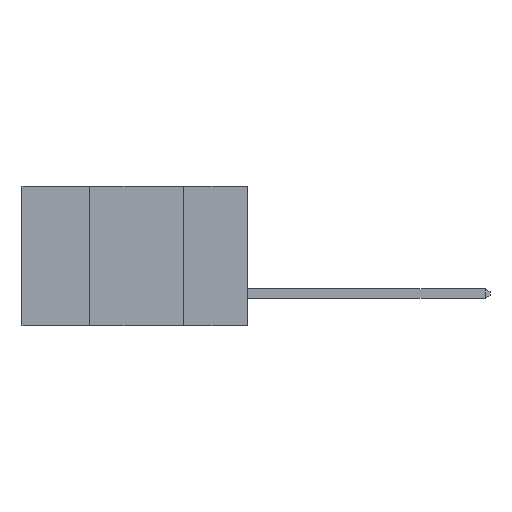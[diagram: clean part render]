
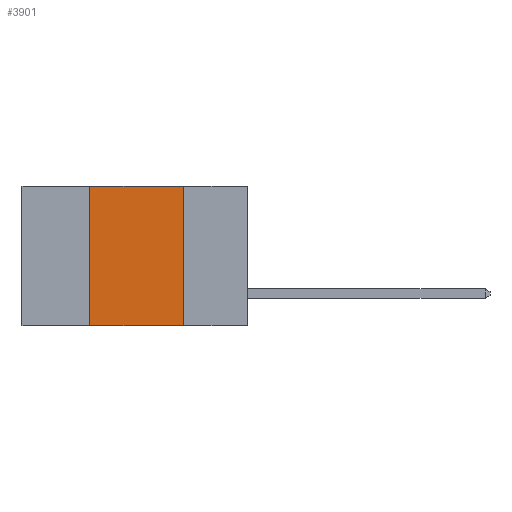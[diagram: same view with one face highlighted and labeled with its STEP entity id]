
A CAD part, left-side view. The second image highlights one B-rep face of the part: STEP entity #3901.
In plain terms, the highlighted planar face has unit normal (-1, 0, 0).
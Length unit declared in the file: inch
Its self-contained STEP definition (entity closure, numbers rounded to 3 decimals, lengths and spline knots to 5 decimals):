
#91 = CARTESIAN_POINT ( 'NONE',  ( 0., 0.6, -0.37 ) ) ;
#471 = CARTESIAN_POINT ( 'NONE',  ( 0., 0.6, 0. ) ) ;
#541 = EDGE_CURVE ( 'NONE', #9583, #4215, #10772, .T. ) ;
#1149 = LINE ( 'NONE', #91, #6142 ) ;
#1496 = ORIENTED_EDGE ( 'NONE', *, *, #4192, .T. ) ;
#2065 = LINE ( 'NONE', #2553, #7037 ) ;
#2484 = VECTOR ( 'NONE', #10289, 39.37008 ) ;
#2553 = CARTESIAN_POINT ( 'NONE',  ( 0., 0.42, 0. ) ) ;
#2764 = VERTEX_POINT ( 'NONE', #6121 ) ;
#2808 = LINE ( 'NONE', #4328, #5478 ) ;
#3460 = CARTESIAN_POINT ( 'NONE',  ( 0., 0.42, 0. ) ) ;
#3813 = EDGE_LOOP ( 'NONE', ( #11535, #6487, #9145, #1496 ) ) ;
#3901 = ADVANCED_FACE ( 'NONE', ( #4592 ), #4044, .F. ) ;
#3959 = AXIS2_PLACEMENT_3D ( 'NONE', #6208, #8726, #5074 ) ;
#4044 = PLANE ( 'NONE',  #3959 ) ;
#4192 = EDGE_CURVE ( 'NONE', #10224, #2764, #1149, .T. ) ;
#4215 = VERTEX_POINT ( 'NONE', #6373 ) ;
#4328 = CARTESIAN_POINT ( 'NONE',  ( 0., 0.17, 0. ) ) ;
#4592 = FACE_OUTER_BOUND ( 'NONE', #3813, .T. ) ;
#5074 = DIRECTION ( 'NONE',  ( 0., 0., -1. ) ) ;
#5137 = DIRECTION ( 'NONE',  ( 0., 0., 1. ) ) ;
#5353 = DIRECTION ( 'NONE',  ( 0., 0., -1. ) ) ;
#5478 = VECTOR ( 'NONE', #5353, 39.37008 ) ;
#6121 = CARTESIAN_POINT ( 'NONE',  ( 0., 0.17, -0.37 ) ) ;
#6142 = VECTOR ( 'NONE', #11161, 39.37008 ) ;
#6208 = CARTESIAN_POINT ( 'NONE',  ( 0., 0.6, 0. ) ) ;
#6373 = CARTESIAN_POINT ( 'NONE',  ( 0., 0.17, 0. ) ) ;
#6487 = ORIENTED_EDGE ( 'NONE', *, *, #541, .F. ) ;
#7037 = VECTOR ( 'NONE', #5137, 39.37008 ) ;
#8726 = DIRECTION ( 'NONE',  ( 1., 0., 0. ) ) ;
#9145 = ORIENTED_EDGE ( 'NONE', *, *, #11090, .F. ) ;
#9583 = VERTEX_POINT ( 'NONE', #3460 ) ;
#10224 = VERTEX_POINT ( 'NONE', #10617 ) ;
#10289 = DIRECTION ( 'NONE',  ( 0., -1., 0. ) ) ;
#10617 = CARTESIAN_POINT ( 'NONE',  ( 0., 0.42, -0.37 ) ) ;
#10772 = LINE ( 'NONE', #471, #2484 ) ;
#11090 = EDGE_CURVE ( 'NONE', #10224, #9583, #2065, .T. ) ;
#11161 = DIRECTION ( 'NONE',  ( 0., -1., 0. ) ) ;
#11243 = EDGE_CURVE ( 'NONE', #4215, #2764, #2808, .T. ) ;
#11535 = ORIENTED_EDGE ( 'NONE', *, *, #11243, .F. ) ;
